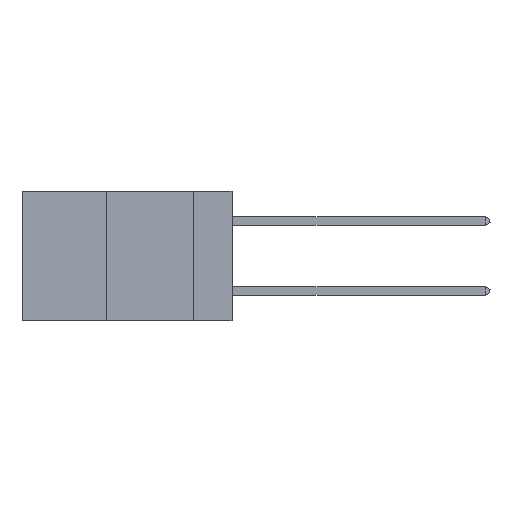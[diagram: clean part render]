
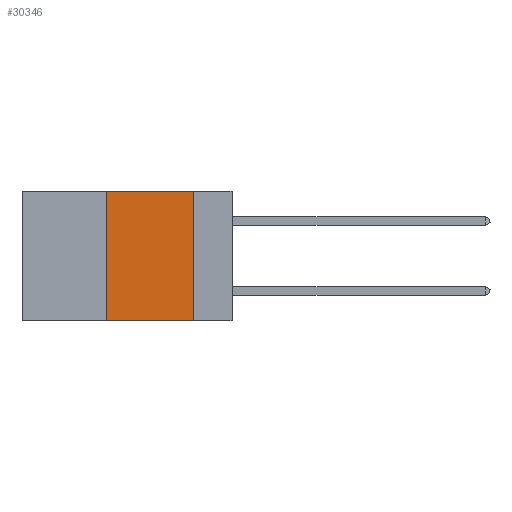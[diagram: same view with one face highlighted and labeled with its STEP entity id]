
A CAD part, left-side view. The second image highlights one B-rep face of the part: STEP entity #30346.
In plain terms, the highlighted planar face has unit normal (-1, 0, 0).
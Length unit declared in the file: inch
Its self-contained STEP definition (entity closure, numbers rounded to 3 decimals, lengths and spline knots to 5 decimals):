
#1355 = LINE ( 'NONE', #16991, #18215 ) ;
#2860 = DIRECTION ( 'NONE',  ( 0., 0., -1. ) ) ;
#3260 = DIRECTION ( 'NONE',  ( 0., -1., 0. ) ) ;
#3558 = CARTESIAN_POINT ( 'NONE',  ( 0., 0.11, -0.37 ) ) ;
#4047 = DIRECTION ( 'NONE',  ( 0., 0., 1. ) ) ;
#7317 = DIRECTION ( 'NONE',  ( 0., 0., -1. ) ) ;
#8185 = DIRECTION ( 'NONE',  ( 0., -1., 0. ) ) ;
#8655 = VERTEX_POINT ( 'NONE', #26797 ) ;
#12856 = VERTEX_POINT ( 'NONE', #18014 ) ;
#13191 = EDGE_CURVE ( 'NONE', #8655, #28157, #29715, .T. ) ;
#14300 = EDGE_CURVE ( 'NONE', #28157, #28266, #27615, .T. ) ;
#14761 = AXIS2_PLACEMENT_3D ( 'NONE', #30832, #20825, #7317 ) ;
#16031 = VECTOR ( 'NONE', #3260, 39.37008 ) ;
#16271 = CARTESIAN_POINT ( 'NONE',  ( 0., 0.11, 0. ) ) ;
#16991 = CARTESIAN_POINT ( 'NONE',  ( 0., 0.36, 0. ) ) ;
#18014 = CARTESIAN_POINT ( 'NONE',  ( 0., 0.36, -0.37 ) ) ;
#18215 = VECTOR ( 'NONE', #4047, 39.37008 ) ;
#18716 = EDGE_CURVE ( 'NONE', #12856, #8655, #1355, .T. ) ;
#20562 = PLANE ( 'NONE',  #14761 ) ;
#20825 = DIRECTION ( 'NONE',  ( 1., 0., 0. ) ) ;
#23816 = VECTOR ( 'NONE', #2860, 39.37008 ) ;
#26557 = EDGE_CURVE ( 'NONE', #12856, #28266, #32027, .T. ) ;
#26797 = CARTESIAN_POINT ( 'NONE',  ( 0., 0.36, 0. ) ) ;
#27615 = LINE ( 'NONE', #16271, #23816 ) ;
#27829 = ORIENTED_EDGE ( 'NONE', *, *, #18716, .F. ) ;
#28157 = VERTEX_POINT ( 'NONE', #43108 ) ;
#28266 = VERTEX_POINT ( 'NONE', #3558 ) ;
#29715 = LINE ( 'NONE', #43376, #16031 ) ;
#30184 = FACE_OUTER_BOUND ( 'NONE', #35957, .T. ) ;
#30346 = ADVANCED_FACE ( 'NONE', ( #30184 ), #20562, .F. ) ;
#30832 = CARTESIAN_POINT ( 'NONE',  ( 0., 0.6, 0. ) ) ;
#31579 = ORIENTED_EDGE ( 'NONE', *, *, #13191, .F. ) ;
#32027 = LINE ( 'NONE', #37943, #34151 ) ;
#34151 = VECTOR ( 'NONE', #8185, 39.37008 ) ;
#34487 = ORIENTED_EDGE ( 'NONE', *, *, #26557, .T. ) ;
#35650 = ORIENTED_EDGE ( 'NONE', *, *, #14300, .F. ) ;
#35957 = EDGE_LOOP ( 'NONE', ( #35650, #31579, #27829, #34487 ) ) ;
#37943 = CARTESIAN_POINT ( 'NONE',  ( 0., 0.6, -0.37 ) ) ;
#43108 = CARTESIAN_POINT ( 'NONE',  ( 0., 0.11, 0. ) ) ;
#43376 = CARTESIAN_POINT ( 'NONE',  ( 0., 0.6, 0. ) ) ;
